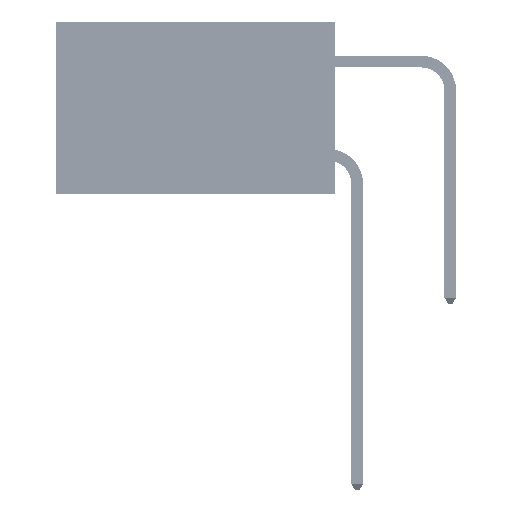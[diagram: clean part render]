
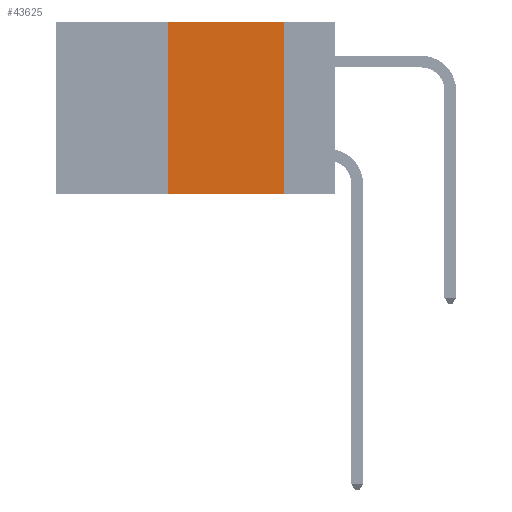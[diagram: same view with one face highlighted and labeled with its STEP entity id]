
A CAD part, left-side view. The second image highlights one B-rep face of the part: STEP entity #43625.
In plain terms, the highlighted planar face has unit normal (-1, 0, 0).
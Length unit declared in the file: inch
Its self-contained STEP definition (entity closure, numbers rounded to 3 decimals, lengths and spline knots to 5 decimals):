
#131 = CARTESIAN_POINT ( 'NONE',  ( 0., 0.36, -0.37 ) ) ;
#471 = LINE ( 'NONE', #16955, #39089 ) ;
#1457 = EDGE_CURVE ( 'NONE', #8123, #23942, #24209, .T. ) ;
#4957 = CARTESIAN_POINT ( 'NONE',  ( 0., 0.36, 0. ) ) ;
#5703 = ORIENTED_EDGE ( 'NONE', *, *, #1457, .F. ) ;
#5928 = VERTEX_POINT ( 'NONE', #131 ) ;
#7412 = FACE_OUTER_BOUND ( 'NONE', #18746, .T. ) ;
#8123 = VERTEX_POINT ( 'NONE', #10046 ) ;
#8611 = EDGE_CURVE ( 'NONE', #27266, #8123, #471, .T. ) ;
#8797 = CARTESIAN_POINT ( 'NONE',  ( 0., 0.6, -0.37 ) ) ;
#10046 = CARTESIAN_POINT ( 'NONE',  ( 0., 0.11, 0. ) ) ;
#10752 = CARTESIAN_POINT ( 'NONE',  ( 0., 0.11, -0.37 ) ) ;
#11177 = DIRECTION ( 'NONE',  ( 0., 0., 1. ) ) ;
#11428 = AXIS2_PLACEMENT_3D ( 'NONE', #34561, #23589, #12813 ) ;
#12638 = EDGE_CURVE ( 'NONE', #5928, #23942, #29150, .T. ) ;
#12813 = DIRECTION ( 'NONE',  ( 0., 0., -1. ) ) ;
#16955 = CARTESIAN_POINT ( 'NONE',  ( 0., 0.6, 0. ) ) ;
#17268 = DIRECTION ( 'NONE',  ( 0., -1., 0. ) ) ;
#17621 = VECTOR ( 'NONE', #34531, 39.37008 ) ;
#18396 = ORIENTED_EDGE ( 'NONE', *, *, #8611, .F. ) ;
#18746 = EDGE_LOOP ( 'NONE', ( #5703, #18396, #41575, #33970 ) ) ;
#19405 = DIRECTION ( 'NONE',  ( 0., 0., -1. ) ) ;
#19585 = LINE ( 'NONE', #32768, #34581 ) ;
#20034 = CARTESIAN_POINT ( 'NONE',  ( 0., 0.11, 0. ) ) ;
#23589 = DIRECTION ( 'NONE',  ( 1., 0., 0. ) ) ;
#23942 = VERTEX_POINT ( 'NONE', #10752 ) ;
#24209 = LINE ( 'NONE', #20034, #32305 ) ;
#27266 = VERTEX_POINT ( 'NONE', #4957 ) ;
#29150 = LINE ( 'NONE', #8797, #17621 ) ;
#32305 = VECTOR ( 'NONE', #19405, 39.37008 ) ;
#32768 = CARTESIAN_POINT ( 'NONE',  ( 0., 0.36, 0. ) ) ;
#33970 = ORIENTED_EDGE ( 'NONE', *, *, #12638, .T. ) ;
#34531 = DIRECTION ( 'NONE',  ( 0., -1., 0. ) ) ;
#34561 = CARTESIAN_POINT ( 'NONE',  ( 0., 0.6, 0. ) ) ;
#34581 = VECTOR ( 'NONE', #11177, 39.37008 ) ;
#34874 = PLANE ( 'NONE',  #11428 ) ;
#39089 = VECTOR ( 'NONE', #17268, 39.37008 ) ;
#41575 = ORIENTED_EDGE ( 'NONE', *, *, #42022, .F. ) ;
#42022 = EDGE_CURVE ( 'NONE', #5928, #27266, #19585, .T. ) ;
#43625 = ADVANCED_FACE ( 'NONE', ( #7412 ), #34874, .F. ) ;
